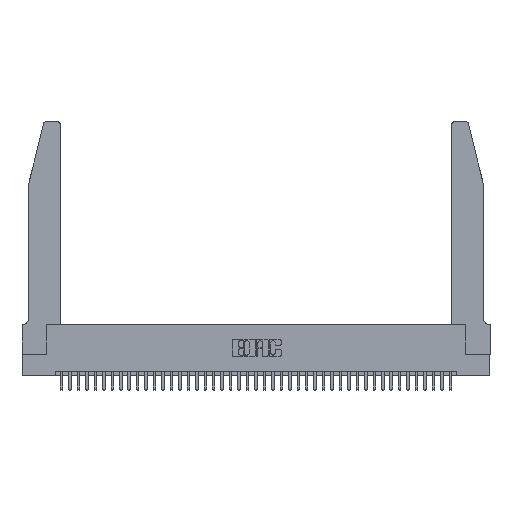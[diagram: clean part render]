
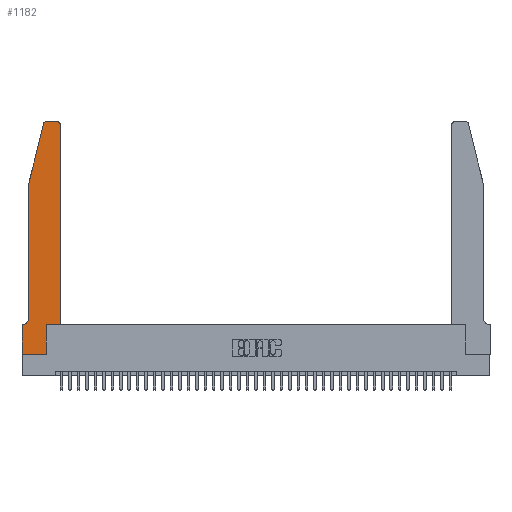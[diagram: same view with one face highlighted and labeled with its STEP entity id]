
A CAD part, top view. The second image highlights one B-rep face of the part: STEP entity #1182.
In plain terms, the highlighted planar face has unit normal (0, 0, 1).
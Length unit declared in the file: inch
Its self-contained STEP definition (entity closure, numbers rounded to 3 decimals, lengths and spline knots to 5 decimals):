
#113 = EDGE_CURVE ( 'NONE', #28582, #39931, #26670, .T. ) ;
#286 = CARTESIAN_POINT ( 'NONE',  ( 0., 0., 0.37 ) ) ;
#528 = CARTESIAN_POINT ( 'NONE',  ( 0.2865, 0.35, 0.37 ) ) ;
#1182 = ADVANCED_FACE ( 'NONE', ( #13193 ), #38718, .T. ) ;
#2950 = VERTEX_POINT ( 'NONE', #25336 ) ;
#3118 = VECTOR ( 'NONE', #40272, 39.37008 ) ;
#3296 = CARTESIAN_POINT ( 'NONE',  ( 0.0755, 2., 0.37 ) ) ;
#3657 = EDGE_CURVE ( 'NONE', #20098, #14718, #23887, .T. ) ;
#3774 = LINE ( 'NONE', #7534, #19635 ) ;
#3844 = DIRECTION ( 'NONE',  ( 1., 0., 0. ) ) ;
#4330 = DIRECTION ( 'NONE',  ( 0., 0., -1. ) ) ;
#5592 = CARTESIAN_POINT ( 'NONE',  ( 0.0755, 2., 0.37 ) ) ;
#6734 = AXIS2_PLACEMENT_3D ( 'NONE', #23305, #4330, #26493 ) ;
#7485 = DIRECTION ( 'NONE',  ( 1., 0., 0. ) ) ;
#7534 = CARTESIAN_POINT ( 'NONE',  ( 0.4505, 0.35, 0.37 ) ) ;
#8149 = AXIS2_PLACEMENT_3D ( 'NONE', #29067, #22828, #3844 ) ;
#8586 = ORIENTED_EDGE ( 'NONE', *, *, #10245, .T. ) ;
#8675 = CARTESIAN_POINT ( 'NONE',  ( 0.0755, 2., 0.37 ) ) ;
#8764 = ORIENTED_EDGE ( 'NONE', *, *, #18338, .T. ) ;
#9076 = CARTESIAN_POINT ( 'NONE',  ( 0.25487, 2.72718, 0.37 ) ) ;
#10245 = EDGE_CURVE ( 'NONE', #39931, #28462, #12682, .T. ) ;
#10718 = DIRECTION ( 'NONE',  ( 0., 1., 0. ) ) ;
#11445 = CARTESIAN_POINT ( 'NONE',  ( 0., 0., 0.37 ) ) ;
#11662 = CARTESIAN_POINT ( 'NONE',  ( 0., 0., 0.37 ) ) ;
#12092 = CARTESIAN_POINT ( 'NONE',  ( 0.4505, 2.72, 0.37 ) ) ;
#12338 = LINE ( 'NONE', #31829, #19747 ) ;
#12560 = LINE ( 'NONE', #11662, #3118 ) ;
#12682 = LINE ( 'NONE', #8675, #21108 ) ;
#12746 = CIRCLE ( 'NONE', #19612, 0.03 ) ;
#13193 = FACE_OUTER_BOUND ( 'NONE', #13654, .T. ) ;
#13215 = EDGE_CURVE ( 'NONE', #14132, #20098, #12746, .T. ) ;
#13361 = VERTEX_POINT ( 'NONE', #11445 ) ;
#13654 = EDGE_LOOP ( 'NONE', ( #29433, #22510, #39300, #8586, #38037, #23112, #8764, #19413, #35838, #25916, #14296, #14283 ) ) ;
#13708 = CARTESIAN_POINT ( 'NONE',  ( 0.4505, 0.35, 0.37 ) ) ;
#13946 = CARTESIAN_POINT ( 'NONE',  ( 0.4205, 2.72, 0.37 ) ) ;
#14132 = VERTEX_POINT ( 'NONE', #12092 ) ;
#14283 = ORIENTED_EDGE ( 'NONE', *, *, #13215, .T. ) ;
#14296 = ORIENTED_EDGE ( 'NONE', *, *, #28326, .T. ) ;
#14522 = VECTOR ( 'NONE', #33602, 39.37008 ) ;
#14578 = CARTESIAN_POINT ( 'NONE',  ( 0.2865, 0.35, 0.37 ) ) ;
#14718 = VERTEX_POINT ( 'NONE', #18006 ) ;
#14759 = VECTOR ( 'NONE', #22433, 39.37008 ) ;
#16122 = DIRECTION ( 'NONE',  ( -0.239, -0.971, 0. ) ) ;
#16191 = LINE ( 'NONE', #13708, #39592 ) ;
#16437 = CIRCLE ( 'NONE', #6734, 0.07 ) ;
#16852 = AXIS2_PLACEMENT_3D ( 'NONE', #18597, #40827, #21783 ) ;
#17131 = DIRECTION ( 'NONE',  ( 1., 0., 0. ) ) ;
#18006 = CARTESIAN_POINT ( 'NONE',  ( 0.284, 2.75, 0.37 ) ) ;
#18338 = EDGE_CURVE ( 'NONE', #32153, #13361, #23133, .T. ) ;
#18519 = EDGE_CURVE ( 'NONE', #32765, #2950, #16191, .T. ) ;
#18597 = CARTESIAN_POINT ( 'NONE',  ( 0.284, 2.72, 0.37 ) ) ;
#19272 = CARTESIAN_POINT ( 'NONE',  ( 0.2865, 0., 0.37 ) ) ;
#19413 = ORIENTED_EDGE ( 'NONE', *, *, #21114, .T. ) ;
#19612 = AXIS2_PLACEMENT_3D ( 'NONE', #13946, #36175, #17131 ) ;
#19635 = VECTOR ( 'NONE', #10718, 39.37008 ) ;
#19736 = CARTESIAN_POINT ( 'NONE',  ( 0.2605, 2.75, 0.37 ) ) ;
#19747 = VECTOR ( 'NONE', #38123, 39.37008 ) ;
#20098 = VERTEX_POINT ( 'NONE', #38404 ) ;
#21108 = VECTOR ( 'NONE', #24443, 39.37008 ) ;
#21114 = EDGE_CURVE ( 'NONE', #13361, #38624, #12560, .T. ) ;
#21783 = DIRECTION ( 'NONE',  ( 1., 0., 0. ) ) ;
#21904 = EDGE_CURVE ( 'NONE', #28462, #36712, #16437, .T. ) ;
#22433 = DIRECTION ( 'NONE',  ( 0., -1., 0. ) ) ;
#22510 = ORIENTED_EDGE ( 'NONE', *, *, #24187, .T. ) ;
#22828 = DIRECTION ( 'NONE',  ( 0., 0., 1. ) ) ;
#22913 = LINE ( 'NONE', #14578, #14522 ) ;
#23112 = ORIENTED_EDGE ( 'NONE', *, *, #34918, .T. ) ;
#23133 = LINE ( 'NONE', #286, #14759 ) ;
#23305 = CARTESIAN_POINT ( 'NONE',  ( 0.0055, 0.42, 0.37 ) ) ;
#23887 = LINE ( 'NONE', #19736, #39850 ) ;
#23929 = CIRCLE ( 'NONE', #16852, 0.03 ) ;
#24187 = EDGE_CURVE ( 'NONE', #14718, #28582, #23929, .T. ) ;
#24443 = DIRECTION ( 'NONE',  ( 0., -1., 0. ) ) ;
#25085 = CARTESIAN_POINT ( 'NONE',  ( 0.0055, 0.35, 0.37 ) ) ;
#25336 = CARTESIAN_POINT ( 'NONE',  ( 0.4505, 0.35, 0.37 ) ) ;
#25916 = ORIENTED_EDGE ( 'NONE', *, *, #18519, .T. ) ;
#25968 = DIRECTION ( 'NONE',  ( -1., 0., 0. ) ) ;
#26493 = DIRECTION ( 'NONE',  ( -1., 0., 0. ) ) ;
#26670 = LINE ( 'NONE', #5592, #33169 ) ;
#28326 = EDGE_CURVE ( 'NONE', #2950, #14132, #3774, .T. ) ;
#28462 = VERTEX_POINT ( 'NONE', #30824 ) ;
#28582 = VERTEX_POINT ( 'NONE', #9076 ) ;
#29067 = CARTESIAN_POINT ( 'NONE',  ( 0., 0.35, 0.37 ) ) ;
#29433 = ORIENTED_EDGE ( 'NONE', *, *, #3657, .T. ) ;
#30824 = CARTESIAN_POINT ( 'NONE',  ( 0.0755, 0.42, 0.37 ) ) ;
#31829 = CARTESIAN_POINT ( 'NONE',  ( 0.0755, 0.35, 0.37 ) ) ;
#31933 = CARTESIAN_POINT ( 'NONE',  ( 0., 0.35, 0.37 ) ) ;
#32153 = VERTEX_POINT ( 'NONE', #31933 ) ;
#32478 = EDGE_CURVE ( 'NONE', #38624, #32765, #22913, .T. ) ;
#32765 = VERTEX_POINT ( 'NONE', #528 ) ;
#33169 = VECTOR ( 'NONE', #16122, 39.37008 ) ;
#33602 = DIRECTION ( 'NONE',  ( 0., 1., 0. ) ) ;
#34918 = EDGE_CURVE ( 'NONE', #36712, #32153, #12338, .T. ) ;
#35838 = ORIENTED_EDGE ( 'NONE', *, *, #32478, .T. ) ;
#36175 = DIRECTION ( 'NONE',  ( 0., 0., 1. ) ) ;
#36712 = VERTEX_POINT ( 'NONE', #25085 ) ;
#38037 = ORIENTED_EDGE ( 'NONE', *, *, #21904, .T. ) ;
#38123 = DIRECTION ( 'NONE',  ( -1., 0., 0. ) ) ;
#38404 = CARTESIAN_POINT ( 'NONE',  ( 0.4205, 2.75, 0.37 ) ) ;
#38624 = VERTEX_POINT ( 'NONE', #19272 ) ;
#38718 = PLANE ( 'NONE',  #8149 ) ;
#39300 = ORIENTED_EDGE ( 'NONE', *, *, #113, .T. ) ;
#39592 = VECTOR ( 'NONE', #7485, 39.37008 ) ;
#39850 = VECTOR ( 'NONE', #25968, 39.37008 ) ;
#39931 = VERTEX_POINT ( 'NONE', #3296 ) ;
#40272 = DIRECTION ( 'NONE',  ( 1., 0., 0. ) ) ;
#40827 = DIRECTION ( 'NONE',  ( 0., 0., 1. ) ) ;
